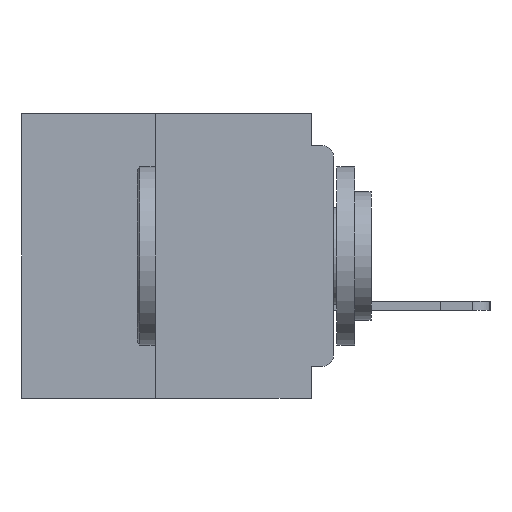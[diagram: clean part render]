
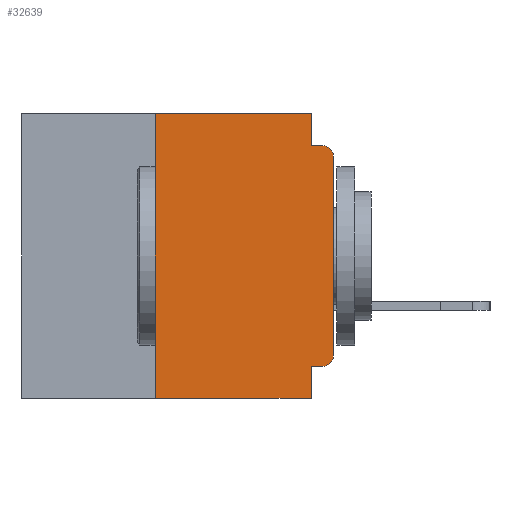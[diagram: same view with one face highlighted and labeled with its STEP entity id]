
A CAD part, left-side view. The second image highlights one B-rep face of the part: STEP entity #32639.
In plain terms, the highlighted planar face has unit normal (-1, 0, 0).
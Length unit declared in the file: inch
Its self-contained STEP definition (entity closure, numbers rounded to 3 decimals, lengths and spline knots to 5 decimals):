
#305 = VERTEX_POINT ( 'NONE', #21332 ) ;
#307 = LINE ( 'NONE', #27357, #15856 ) ;
#448 = LINE ( 'NONE', #21280, #32449 ) ;
#718 = CARTESIAN_POINT ( 'NONE',  ( 0., 0.437, -0.4 ) ) ;
#1255 = EDGE_CURVE ( 'NONE', #7222, #305, #307, .T. ) ;
#1914 = CARTESIAN_POINT ( 'NONE',  ( 0., 0.437, 0. ) ) ;
#2655 = AXIS2_PLACEMENT_3D ( 'NONE', #22179, #3546, #25276 ) ;
#3232 = EDGE_CURVE ( 'NONE', #19814, #7222, #12253, .T. ) ;
#3546 = DIRECTION ( 'NONE',  ( -1., 0., 0. ) ) ;
#4021 = VECTOR ( 'NONE', #34187, 39.37008 ) ;
#5163 = DIRECTION ( 'NONE',  ( 1., 0., 0. ) ) ;
#6023 = CARTESIAN_POINT ( 'NONE',  ( 0., 0.031, -0.4 ) ) ;
#6442 = LINE ( 'NONE', #6023, #37415 ) ;
#6518 = EDGE_CURVE ( 'NONE', #305, #8469, #23863, .T. ) ;
#7066 = CARTESIAN_POINT ( 'NONE',  ( 0., 0., -0.06 ) ) ;
#7222 = VERTEX_POINT ( 'NONE', #18677 ) ;
#7980 = ORIENTED_EDGE ( 'NONE', *, *, #39091, .T. ) ;
#8469 = VERTEX_POINT ( 'NONE', #12933 ) ;
#9084 = DIRECTION ( 'NONE',  ( 0., 0., 1. ) ) ;
#9567 = ORIENTED_EDGE ( 'NONE', *, *, #26346, .T. ) ;
#9593 = DIRECTION ( 'NONE',  ( -1., 0., 0. ) ) ;
#9626 = ORIENTED_EDGE ( 'NONE', *, *, #26238, .F. ) ;
#10391 = VERTEX_POINT ( 'NONE', #17213 ) ;
#10680 = EDGE_LOOP ( 'NONE', ( #7980, #9567, #9626, #15222, #14269, #31304, #31963, #25721, #23878, #39720 ) ) ;
#12071 = CIRCLE ( 'NONE', #16519, 0.015 ) ;
#12253 = LINE ( 'NONE', #33618, #4021 ) ;
#12354 = DIRECTION ( 'NONE',  ( 0., 1., 0. ) ) ;
#12707 = VECTOR ( 'NONE', #9084, 39.37008 ) ;
#12933 = CARTESIAN_POINT ( 'NONE',  ( 0., 0.031, -0.045 ) ) ;
#13629 = EDGE_CURVE ( 'NONE', #39427, #37106, #6442, .T. ) ;
#13820 = VERTEX_POINT ( 'NONE', #7066 ) ;
#14269 = ORIENTED_EDGE ( 'NONE', *, *, #1255, .F. ) ;
#14565 = DIRECTION ( 'NONE',  ( 0., -1., 0. ) ) ;
#15222 = ORIENTED_EDGE ( 'NONE', *, *, #6518, .F. ) ;
#15411 = DIRECTION ( 'NONE',  ( 0., 0., -1. ) ) ;
#15571 = VECTOR ( 'NONE', #30703, 39.37008 ) ;
#15583 = CARTESIAN_POINT ( 'NONE',  ( 0., 0.015, -0.045 ) ) ;
#15856 = VECTOR ( 'NONE', #14565, 39.37008 ) ;
#16519 = AXIS2_PLACEMENT_3D ( 'NONE', #28235, #9593, #31308 ) ;
#16678 = CIRCLE ( 'NONE', #2655, 0.015 ) ;
#17213 = CARTESIAN_POINT ( 'NONE',  ( 0., 0.015, -0.355 ) ) ;
#17628 = CARTESIAN_POINT ( 'NONE',  ( 0., 0.25, -0.4 ) ) ;
#18154 = DIRECTION ( 'NONE',  ( 0., -1., 0. ) ) ;
#18389 = EDGE_CURVE ( 'NONE', #19814, #37106, #21823, .T. ) ;
#18659 = CARTESIAN_POINT ( 'NONE',  ( 0., 0.031, -0.4 ) ) ;
#18677 = CARTESIAN_POINT ( 'NONE',  ( 0., 0.25, 0. ) ) ;
#19814 = VERTEX_POINT ( 'NONE', #17628 ) ;
#20861 = VECTOR ( 'NONE', #25566, 39.37008 ) ;
#20889 = VECTOR ( 'NONE', #12354, 39.37008 ) ;
#21015 = CARTESIAN_POINT ( 'NONE',  ( 0., 0., -0.34 ) ) ;
#21057 = LINE ( 'NONE', #36683, #12707 ) ;
#21174 = CARTESIAN_POINT ( 'NONE',  ( 0., 0.031, 0. ) ) ;
#21280 = CARTESIAN_POINT ( 'NONE',  ( 0., 0., -0.045 ) ) ;
#21332 = CARTESIAN_POINT ( 'NONE',  ( 0., 0.031, 0. ) ) ;
#21639 = VERTEX_POINT ( 'NONE', #21015 ) ;
#21823 = LINE ( 'NONE', #718, #20861 ) ;
#21853 = LINE ( 'NONE', #30927, #20889 ) ;
#22179 = CARTESIAN_POINT ( 'NONE',  ( 0., 0.015, -0.34 ) ) ;
#23115 = CARTESIAN_POINT ( 'NONE',  ( 0., 0.031, -0.355 ) ) ;
#23789 = PLANE ( 'NONE',  #37694 ) ;
#23863 = LINE ( 'NONE', #21174, #15571 ) ;
#23878 = ORIENTED_EDGE ( 'NONE', *, *, #29255, .F. ) ;
#24993 = FACE_OUTER_BOUND ( 'NONE', #10680, .T. ) ;
#25276 = DIRECTION ( 'NONE',  ( 0., 0., -1. ) ) ;
#25566 = DIRECTION ( 'NONE',  ( 0., -1., 0. ) ) ;
#25721 = ORIENTED_EDGE ( 'NONE', *, *, #13629, .F. ) ;
#26238 = EDGE_CURVE ( 'NONE', #8469, #26926, #448, .T. ) ;
#26346 = EDGE_CURVE ( 'NONE', #13820, #26926, #12071, .T. ) ;
#26884 = DIRECTION ( 'NONE',  ( 0., 0., -1. ) ) ;
#26926 = VERTEX_POINT ( 'NONE', #15583 ) ;
#27357 = CARTESIAN_POINT ( 'NONE',  ( 0., 0.437, 0. ) ) ;
#28235 = CARTESIAN_POINT ( 'NONE',  ( 0., 0.015, -0.06 ) ) ;
#29255 = EDGE_CURVE ( 'NONE', #10391, #39427, #21853, .T. ) ;
#30703 = DIRECTION ( 'NONE',  ( 0., 0., -1. ) ) ;
#30927 = CARTESIAN_POINT ( 'NONE',  ( 0., 0., -0.355 ) ) ;
#31304 = ORIENTED_EDGE ( 'NONE', *, *, #3232, .F. ) ;
#31308 = DIRECTION ( 'NONE',  ( 0., 0., -1. ) ) ;
#31963 = ORIENTED_EDGE ( 'NONE', *, *, #18389, .T. ) ;
#32449 = VECTOR ( 'NONE', #18154, 39.37008 ) ;
#32639 = ADVANCED_FACE ( 'NONE', ( #24993 ), #23789, .F. ) ;
#33618 = CARTESIAN_POINT ( 'NONE',  ( 0., 0.25, -0.4 ) ) ;
#34187 = DIRECTION ( 'NONE',  ( 0., 0., 1. ) ) ;
#36683 = CARTESIAN_POINT ( 'NONE',  ( 0., 0., 0. ) ) ;
#37106 = VERTEX_POINT ( 'NONE', #18659 ) ;
#37415 = VECTOR ( 'NONE', #15411, 39.37008 ) ;
#37694 = AXIS2_PLACEMENT_3D ( 'NONE', #1914, #5163, #26884 ) ;
#38607 = EDGE_CURVE ( 'NONE', #10391, #21639, #16678, .T. ) ;
#39091 = EDGE_CURVE ( 'NONE', #21639, #13820, #21057, .T. ) ;
#39427 = VERTEX_POINT ( 'NONE', #23115 ) ;
#39720 = ORIENTED_EDGE ( 'NONE', *, *, #38607, .T. ) ;
